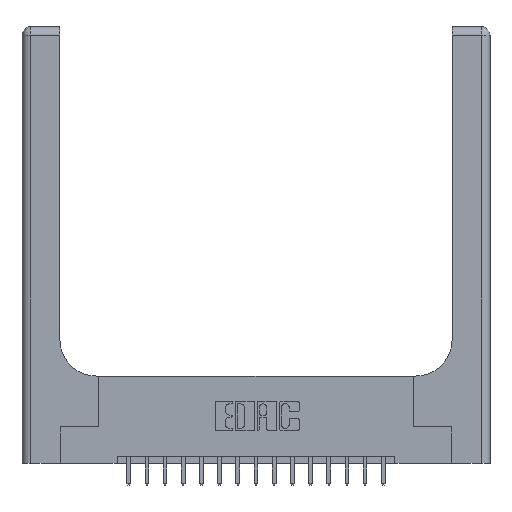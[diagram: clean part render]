
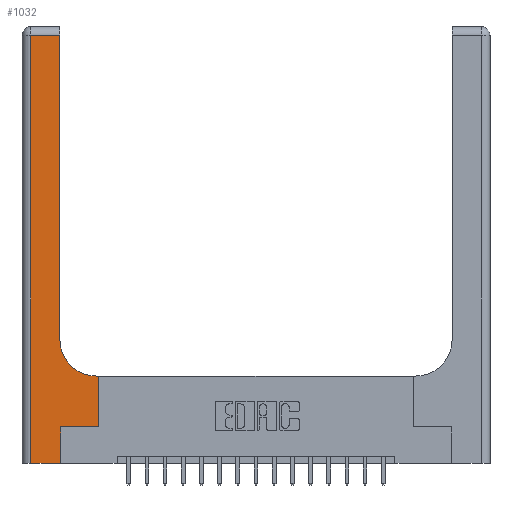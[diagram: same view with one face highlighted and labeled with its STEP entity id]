
A CAD part, top view. The second image highlights one B-rep face of the part: STEP entity #1032.
In plain terms, the highlighted planar face has unit normal (0, 0, 1).
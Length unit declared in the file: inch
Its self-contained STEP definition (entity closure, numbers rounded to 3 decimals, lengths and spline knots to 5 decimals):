
#90 = FACE_OUTER_BOUND ( 'NONE', #15017, .T. ) ;
#230 = ORIENTED_EDGE ( 'NONE', *, *, #7430, .T. ) ;
#374 = CARTESIAN_POINT ( 'NONE',  ( 0.06, 3., 0.37 ) ) ;
#494 = CARTESIAN_POINT ( 'NONE',  ( 0.51, 0.85, 0.37 ) ) ;
#550 = DIRECTION ( 'NONE',  ( -1., 0., 0. ) ) ;
#1032 = ADVANCED_FACE ( 'NONE', ( #90 ), #14678, .F. ) ;
#1454 = CARTESIAN_POINT ( 'NONE',  ( 0., 2.94, 0.37 ) ) ;
#1706 = EDGE_CURVE ( 'NONE', #13823, #17735, #14737, .T. ) ;
#1715 = DIRECTION ( 'NONE',  ( 0., -1., 0. ) ) ;
#1997 = ORIENTED_EDGE ( 'NONE', *, *, #3811, .T. ) ;
#2465 = EDGE_CURVE ( 'NONE', #17735, #7609, #2515, .T. ) ;
#2515 = LINE ( 'NONE', #9890, #5698 ) ;
#2646 = ORIENTED_EDGE ( 'NONE', *, *, #14842, .T. ) ;
#3251 = ORIENTED_EDGE ( 'NONE', *, *, #7012, .T. ) ;
#3434 = CARTESIAN_POINT ( 'NONE',  ( 0.265, 0., 0.37 ) ) ;
#3529 = DIRECTION ( 'NONE',  ( 1., 0., 0. ) ) ;
#3757 = VERTEX_POINT ( 'NONE', #16053 ) ;
#3811 = EDGE_CURVE ( 'NONE', #8523, #6951, #12634, .T. ) ;
#5376 = VERTEX_POINT ( 'NONE', #7308 ) ;
#5447 = ORIENTED_EDGE ( 'NONE', *, *, #8863, .T. ) ;
#5698 = VECTOR ( 'NONE', #15792, 39.37008 ) ;
#5941 = DIRECTION ( 'NONE',  ( 1., 0., 0. ) ) ;
#6083 = CARTESIAN_POINT ( 'NONE',  ( 0.265, 0.25, 0.37 ) ) ;
#6579 = LINE ( 'NONE', #6656, #8381 ) ;
#6656 = CARTESIAN_POINT ( 'NONE',  ( 0.26, 3., 0.37 ) ) ;
#6878 = AXIS2_PLACEMENT_3D ( 'NONE', #494, #13270, #11899 ) ;
#6951 = VERTEX_POINT ( 'NONE', #11650 ) ;
#7012 = EDGE_CURVE ( 'NONE', #6951, #18581, #11372, .T. ) ;
#7308 = CARTESIAN_POINT ( 'NONE',  ( 0.26, 0.85, 0.37 ) ) ;
#7392 = CARTESIAN_POINT ( 'NONE',  ( 0.265, 0.25, 0.37 ) ) ;
#7430 = EDGE_CURVE ( 'NONE', #7609, #3757, #10706, .T. ) ;
#7563 = VECTOR ( 'NONE', #3529, 39.37008 ) ;
#7609 = VERTEX_POINT ( 'NONE', #12979 ) ;
#7886 = AXIS2_PLACEMENT_3D ( 'NONE', #16096, #17515, #8939 ) ;
#8381 = VECTOR ( 'NONE', #13893, 39.37008 ) ;
#8523 = VERTEX_POINT ( 'NONE', #10290 ) ;
#8863 = EDGE_CURVE ( 'NONE', #16469, #8523, #16264, .T. ) ;
#8939 = DIRECTION ( 'NONE',  ( -1., 0., 0. ) ) ;
#9890 = CARTESIAN_POINT ( 'NONE',  ( 0.528, 0.25, 0.37 ) ) ;
#9964 = VECTOR ( 'NONE', #15294, 39.37008 ) ;
#10290 = CARTESIAN_POINT ( 'NONE',  ( 0.06, 2.94, 0.37 ) ) ;
#10706 = LINE ( 'NONE', #15172, #13160 ) ;
#11372 = LINE ( 'NONE', #14940, #7563 ) ;
#11650 = CARTESIAN_POINT ( 'NONE',  ( 0.06, 0., 0.37 ) ) ;
#11835 = ORIENTED_EDGE ( 'NONE', *, *, #14806, .T. ) ;
#11899 = DIRECTION ( 'NONE',  ( 1., 0., 0. ) ) ;
#12213 = VECTOR ( 'NONE', #550, 39.37008 ) ;
#12634 = LINE ( 'NONE', #374, #14666 ) ;
#12751 = ORIENTED_EDGE ( 'NONE', *, *, #2465, .T. ) ;
#12782 = CARTESIAN_POINT ( 'NONE',  ( 0.26, 2.94, 0.37 ) ) ;
#12834 = EDGE_CURVE ( 'NONE', #3757, #5376, #17016, .T. ) ;
#12979 = CARTESIAN_POINT ( 'NONE',  ( 0.528, 0.6, 0.37 ) ) ;
#13160 = VECTOR ( 'NONE', #14984, 39.37008 ) ;
#13270 = DIRECTION ( 'NONE',  ( 0., 0., -1. ) ) ;
#13779 = LINE ( 'NONE', #13957, #9964 ) ;
#13823 = VERTEX_POINT ( 'NONE', #6083 ) ;
#13893 = DIRECTION ( 'NONE',  ( 0., 1., 0. ) ) ;
#13957 = CARTESIAN_POINT ( 'NONE',  ( 0.265, 0., 0.37 ) ) ;
#14560 = ORIENTED_EDGE ( 'NONE', *, *, #1706, .T. ) ;
#14666 = VECTOR ( 'NONE', #1715, 39.37008 ) ;
#14678 = PLANE ( 'NONE',  #7886 ) ;
#14737 = LINE ( 'NONE', #7392, #17612 ) ;
#14806 = EDGE_CURVE ( 'NONE', #18581, #13823, #13779, .T. ) ;
#14842 = EDGE_CURVE ( 'NONE', #5376, #16469, #6579, .T. ) ;
#14940 = CARTESIAN_POINT ( 'NONE',  ( 0., 0., 0.37 ) ) ;
#14984 = DIRECTION ( 'NONE',  ( -1., 0., 0. ) ) ;
#15017 = EDGE_LOOP ( 'NONE', ( #2646, #5447, #1997, #3251, #11835, #14560, #12751, #230, #15254 ) ) ;
#15172 = CARTESIAN_POINT ( 'NONE',  ( 0.26, 0.6, 0.37 ) ) ;
#15254 = ORIENTED_EDGE ( 'NONE', *, *, #12834, .T. ) ;
#15294 = DIRECTION ( 'NONE',  ( 0., 1., 0. ) ) ;
#15792 = DIRECTION ( 'NONE',  ( 0., 1., 0. ) ) ;
#16053 = CARTESIAN_POINT ( 'NONE',  ( 0.51, 0.6, 0.37 ) ) ;
#16096 = CARTESIAN_POINT ( 'NONE',  ( 0., 3., 0.37 ) ) ;
#16264 = LINE ( 'NONE', #1454, #12213 ) ;
#16469 = VERTEX_POINT ( 'NONE', #12782 ) ;
#17016 = CIRCLE ( 'NONE', #6878, 0.25 ) ;
#17238 = CARTESIAN_POINT ( 'NONE',  ( 0.528, 0.25, 0.37 ) ) ;
#17515 = DIRECTION ( 'NONE',  ( 0., 0., -1. ) ) ;
#17612 = VECTOR ( 'NONE', #5941, 39.37008 ) ;
#17735 = VERTEX_POINT ( 'NONE', #17238 ) ;
#18581 = VERTEX_POINT ( 'NONE', #3434 ) ;
